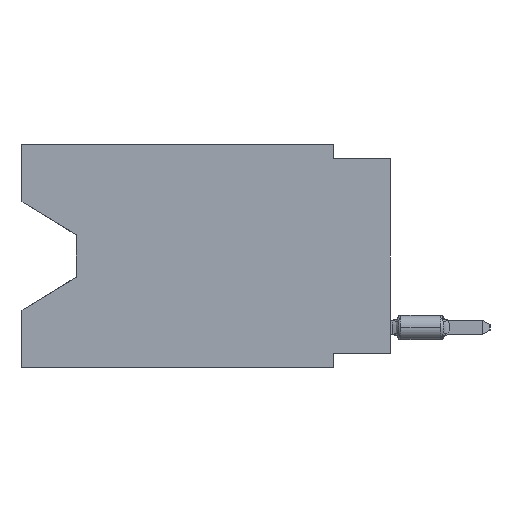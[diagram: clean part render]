
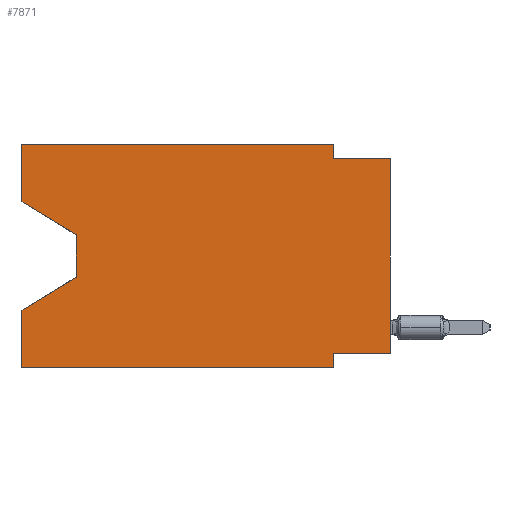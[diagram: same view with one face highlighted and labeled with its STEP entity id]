
A CAD part, left-side view. The second image highlights one B-rep face of the part: STEP entity #7871.
In plain terms, the highlighted planar face has unit normal (-1, 0, 0).
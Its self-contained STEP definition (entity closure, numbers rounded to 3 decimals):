
#299 = EDGE_CURVE ( 'NONE', #18376, #27117, #29147, .T. ) ;
#1194 = CARTESIAN_POINT ( 'NONE',  ( 0., 13.97, -5.893 ) ) ;
#1714 = ORIENTED_EDGE ( 'NONE', *, *, #9803, .T. ) ;
#1922 = VECTOR ( 'NONE', #22032, 1000. ) ;
#2027 = CARTESIAN_POINT ( 'NONE',  ( 0., 2.54, -9.906 ) ) ;
#2078 = LINE ( 'NONE', #18904, #18141 ) ;
#2141 = CARTESIAN_POINT ( 'NONE',  ( 0., 2.54, 0. ) ) ;
#2232 = VERTEX_POINT ( 'NONE', #27276 ) ;
#2855 = ORIENTED_EDGE ( 'NONE', *, *, #20733, .F. ) ;
#3096 = DIRECTION ( 'NONE',  ( 0., -1., 0. ) ) ;
#3474 = DIRECTION ( 'NONE',  ( 0., 0.855, -0.519 ) ) ;
#4108 = CARTESIAN_POINT ( 'NONE',  ( 0., 16.383, -7.36 ) ) ;
#4362 = EDGE_CURVE ( 'NONE', #26560, #28908, #21392, .T. ) ;
#5680 = LINE ( 'NONE', #8425, #15740 ) ;
#5850 = VERTEX_POINT ( 'NONE', #11986 ) ;
#5896 = PLANE ( 'NONE',  #18220 ) ;
#6307 = EDGE_CURVE ( 'NONE', #18855, #13326, #14061, .T. ) ;
#6865 = EDGE_LOOP ( 'NONE', ( #20582, #24359, #1714, #30284, #7272, #15730, #28823, #25961, #14412, #2855, #25622, #8097 ) ) ;
#7014 = EDGE_CURVE ( 'NONE', #18855, #18376, #24793, .T. ) ;
#7272 = ORIENTED_EDGE ( 'NONE', *, *, #10176, .T. ) ;
#7871 = ADVANCED_FACE ( 'NONE', ( #23543 ), #5896, .F. ) ;
#8097 = ORIENTED_EDGE ( 'NONE', *, *, #7014, .F. ) ;
#8425 = CARTESIAN_POINT ( 'NONE',  ( 0., 16.383, -9.906 ) ) ;
#8489 = DIRECTION ( 'NONE',  ( 1., 0., 0. ) ) ;
#8869 = VECTOR ( 'NONE', #12817, 1000. ) ;
#9470 = DIRECTION ( 'NONE',  ( 0., 0., 1. ) ) ;
#9764 = DIRECTION ( 'NONE',  ( 0., 0., -1. ) ) ;
#9803 = EDGE_CURVE ( 'NONE', #2232, #20162, #27890, .T. ) ;
#10008 = CARTESIAN_POINT ( 'NONE',  ( 0., 0., -9.271 ) ) ;
#10176 = EDGE_CURVE ( 'NONE', #29447, #24195, #5680, .T. ) ;
#10537 = CARTESIAN_POINT ( 'NONE',  ( 0., 16.383, -2.546 ) ) ;
#10919 = CARTESIAN_POINT ( 'NONE',  ( 0., 16.383, 0. ) ) ;
#11637 = CARTESIAN_POINT ( 'NONE',  ( 0., 16.383, -2.546 ) ) ;
#11986 = CARTESIAN_POINT ( 'NONE',  ( 0., 0., -9.271 ) ) ;
#12214 = CARTESIAN_POINT ( 'NONE',  ( 0., 0., -0.635 ) ) ;
#12817 = DIRECTION ( 'NONE',  ( 0., 0., 1. ) ) ;
#13326 = VERTEX_POINT ( 'NONE', #15987 ) ;
#13468 = EDGE_CURVE ( 'NONE', #24395, #24195, #26918, .T. ) ;
#14061 = LINE ( 'NONE', #11637, #20426 ) ;
#14374 = CARTESIAN_POINT ( 'NONE',  ( 0., 16.383, 0. ) ) ;
#14412 = ORIENTED_EDGE ( 'NONE', *, *, #4362, .F. ) ;
#15188 = VECTOR ( 'NONE', #3474, 1000. ) ;
#15604 = DIRECTION ( 'NONE',  ( 0., 0., -1. ) ) ;
#15730 = ORIENTED_EDGE ( 'NONE', *, *, #13468, .F. ) ;
#15740 = VECTOR ( 'NONE', #3096, 1000. ) ;
#15877 = CARTESIAN_POINT ( 'NONE',  ( 0., 16.383, -9.906 ) ) ;
#15987 = CARTESIAN_POINT ( 'NONE',  ( 0., 13.97, -4.013 ) ) ;
#16243 = VECTOR ( 'NONE', #9764, 1000. ) ;
#16362 = VECTOR ( 'NONE', #17953, 1000. ) ;
#16758 = LINE ( 'NONE', #26631, #31393 ) ;
#17469 = CARTESIAN_POINT ( 'NONE',  ( 0., 2.54, 0. ) ) ;
#17953 = DIRECTION ( 'NONE',  ( 0., 0., -1. ) ) ;
#18107 = EDGE_CURVE ( 'NONE', #5850, #24395, #29922, .T. ) ;
#18141 = VECTOR ( 'NONE', #21018, 1000. ) ;
#18220 = AXIS2_PLACEMENT_3D ( 'NONE', #10919, #8489, #15604 ) ;
#18376 = VERTEX_POINT ( 'NONE', #14374 ) ;
#18855 = VERTEX_POINT ( 'NONE', #10537 ) ;
#18904 = CARTESIAN_POINT ( 'NONE',  ( 0., 16.383, 0. ) ) ;
#19127 = CARTESIAN_POINT ( 'NONE',  ( 0., 16.383, 0. ) ) ;
#19893 = DIRECTION ( 'NONE',  ( 0., 1., 0. ) ) ;
#20144 = VECTOR ( 'NONE', #21767, 1000. ) ;
#20162 = VERTEX_POINT ( 'NONE', #4108 ) ;
#20426 = VECTOR ( 'NONE', #27099, 1000. ) ;
#20582 = ORIENTED_EDGE ( 'NONE', *, *, #6307, .T. ) ;
#20733 = EDGE_CURVE ( 'NONE', #27117, #26560, #30425, .T. ) ;
#21018 = DIRECTION ( 'NONE',  ( 0., 0., 1. ) ) ;
#21392 = LINE ( 'NONE', #23834, #28297 ) ;
#21767 = DIRECTION ( 'NONE',  ( 0., 0., -1. ) ) ;
#21915 = CARTESIAN_POINT ( 'NONE',  ( 0., 13.97, -4.013 ) ) ;
#22032 = DIRECTION ( 'NONE',  ( 0., -1., 0. ) ) ;
#22211 = CARTESIAN_POINT ( 'NONE',  ( 0., 16.383, 0. ) ) ;
#22805 = CARTESIAN_POINT ( 'NONE',  ( 0., 2.54, -9.271 ) ) ;
#23543 = FACE_OUTER_BOUND ( 'NONE', #6865, .T. ) ;
#23834 = CARTESIAN_POINT ( 'NONE',  ( 0., 0., -0.635 ) ) ;
#24195 = VERTEX_POINT ( 'NONE', #25584 ) ;
#24359 = ORIENTED_EDGE ( 'NONE', *, *, #28960, .T. ) ;
#24395 = VERTEX_POINT ( 'NONE', #22805 ) ;
#24793 = LINE ( 'NONE', #22211, #8869 ) ;
#25034 = EDGE_CURVE ( 'NONE', #5850, #28908, #16758, .T. ) ;
#25584 = CARTESIAN_POINT ( 'NONE',  ( 0., 2.54, -9.906 ) ) ;
#25622 = ORIENTED_EDGE ( 'NONE', *, *, #299, .F. ) ;
#25961 = ORIENTED_EDGE ( 'NONE', *, *, #25034, .T. ) ;
#26560 = VERTEX_POINT ( 'NONE', #31617 ) ;
#26631 = CARTESIAN_POINT ( 'NONE',  ( 0., 0., 0. ) ) ;
#26918 = LINE ( 'NONE', #2027, #16243 ) ;
#27099 = DIRECTION ( 'NONE',  ( 0., -0.855, -0.519 ) ) ;
#27117 = VERTEX_POINT ( 'NONE', #2141 ) ;
#27276 = CARTESIAN_POINT ( 'NONE',  ( 0., 13.97, -5.893 ) ) ;
#27890 = LINE ( 'NONE', #1194, #15188 ) ;
#28297 = VECTOR ( 'NONE', #30963, 1000. ) ;
#28365 = EDGE_CURVE ( 'NONE', #29447, #20162, #2078, .T. ) ;
#28823 = ORIENTED_EDGE ( 'NONE', *, *, #18107, .F. ) ;
#28908 = VERTEX_POINT ( 'NONE', #12214 ) ;
#28960 = EDGE_CURVE ( 'NONE', #13326, #2232, #29842, .T. ) ;
#29147 = LINE ( 'NONE', #19127, #1922 ) ;
#29447 = VERTEX_POINT ( 'NONE', #15877 ) ;
#29842 = LINE ( 'NONE', #21915, #20144 ) ;
#29922 = LINE ( 'NONE', #10008, #30741 ) ;
#30284 = ORIENTED_EDGE ( 'NONE', *, *, #28365, .F. ) ;
#30425 = LINE ( 'NONE', #17469, #16362 ) ;
#30741 = VECTOR ( 'NONE', #19893, 1000. ) ;
#30963 = DIRECTION ( 'NONE',  ( 0., -1., 0. ) ) ;
#31393 = VECTOR ( 'NONE', #9470, 1000. ) ;
#31617 = CARTESIAN_POINT ( 'NONE',  ( 0., 2.54, -0.635 ) ) ;
